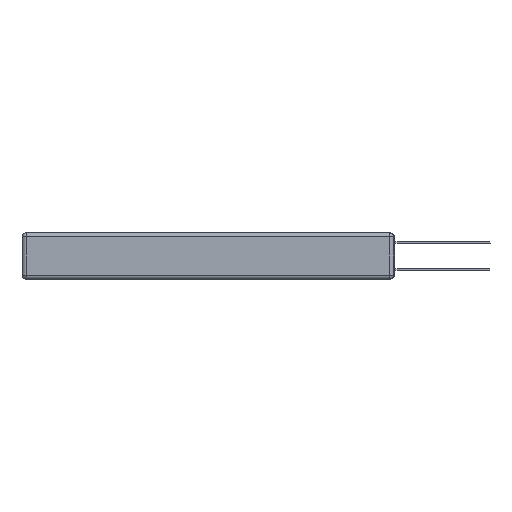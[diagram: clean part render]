
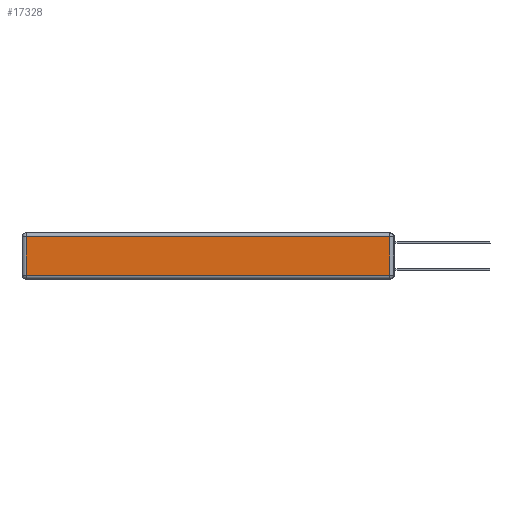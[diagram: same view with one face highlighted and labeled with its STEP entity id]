
A CAD part, left-side view. The second image highlights one B-rep face of the part: STEP entity #17328.
In plain terms, the highlighted planar face has unit normal (-1, 0, 0).
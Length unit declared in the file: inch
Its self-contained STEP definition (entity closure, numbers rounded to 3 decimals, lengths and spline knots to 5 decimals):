
#150 = FACE_OUTER_BOUND ( 'NONE', #19891, .T. ) ;
#1927 = CARTESIAN_POINT ( 'NONE',  ( 0., 2.72, -0.313 ) ) ;
#2974 = EDGE_CURVE ( 'NONE', #13722, #11288, #8699, .T. ) ;
#3139 = DIRECTION ( 'NONE',  ( 0., 0., -1. ) ) ;
#5842 = LINE ( 'NONE', #20464, #13694 ) ;
#5950 = ORIENTED_EDGE ( 'NONE', *, *, #2974, .T. ) ;
#6888 = CARTESIAN_POINT ( 'NONE',  ( 0., 2.72, -0.343 ) ) ;
#7303 = DIRECTION ( 'NONE',  ( 0., -1., 0. ) ) ;
#8023 = ORIENTED_EDGE ( 'NONE', *, *, #22107, .T. ) ;
#8699 = LINE ( 'NONE', #6888, #10066 ) ;
#10066 = VECTOR ( 'NONE', #3139, 39.37008 ) ;
#10926 = DIRECTION ( 'NONE',  ( -1., 0., 0. ) ) ;
#11288 = VERTEX_POINT ( 'NONE', #1927 ) ;
#12909 = VECTOR ( 'NONE', #15313, 39.37008 ) ;
#12999 = PLANE ( 'NONE',  #16146 ) ;
#13025 = CARTESIAN_POINT ( 'NONE',  ( 0., 0., -0.313 ) ) ;
#13484 = DIRECTION ( 'NONE',  ( 0., 0., 1. ) ) ;
#13694 = VECTOR ( 'NONE', #13484, 39.37008 ) ;
#13722 = VERTEX_POINT ( 'NONE', #15360 ) ;
#14407 = EDGE_CURVE ( 'NONE', #15954, #22197, #5842, .T. ) ;
#14834 = LINE ( 'NONE', #13025, #16800 ) ;
#15313 = DIRECTION ( 'NONE',  ( 0., 1., 0. ) ) ;
#15360 = CARTESIAN_POINT ( 'NONE',  ( 0., 2.72, -0.03 ) ) ;
#15954 = VERTEX_POINT ( 'NONE', #23603 ) ;
#16146 = AXIS2_PLACEMENT_3D ( 'NONE', #19958, #10926, #16643 ) ;
#16643 = DIRECTION ( 'NONE',  ( 0., 0., 1. ) ) ;
#16800 = VECTOR ( 'NONE', #7303, 39.37008 ) ;
#17328 = ADVANCED_FACE ( 'NONE', ( #150 ), #12999, .T. ) ;
#17382 = LINE ( 'NONE', #20578, #12909 ) ;
#17385 = CARTESIAN_POINT ( 'NONE',  ( 0., 0.03, -0.03 ) ) ;
#18155 = ORIENTED_EDGE ( 'NONE', *, *, #20969, .T. ) ;
#19891 = EDGE_LOOP ( 'NONE', ( #8023, #23637, #18155, #5950 ) ) ;
#19958 = CARTESIAN_POINT ( 'NONE',  ( 0., 0., -0.343 ) ) ;
#20464 = CARTESIAN_POINT ( 'NONE',  ( 0., 0.03, -0.343 ) ) ;
#20578 = CARTESIAN_POINT ( 'NONE',  ( 0., 2.75, -0.03 ) ) ;
#20969 = EDGE_CURVE ( 'NONE', #22197, #13722, #17382, .T. ) ;
#22107 = EDGE_CURVE ( 'NONE', #11288, #15954, #14834, .T. ) ;
#22197 = VERTEX_POINT ( 'NONE', #17385 ) ;
#23603 = CARTESIAN_POINT ( 'NONE',  ( 0., 0.03, -0.313 ) ) ;
#23637 = ORIENTED_EDGE ( 'NONE', *, *, #14407, .T. ) ;
